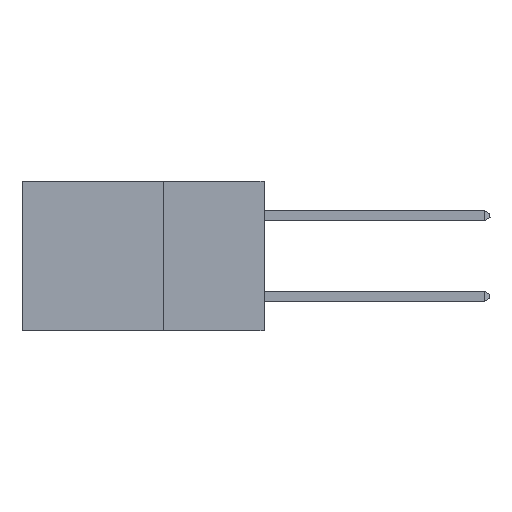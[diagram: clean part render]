
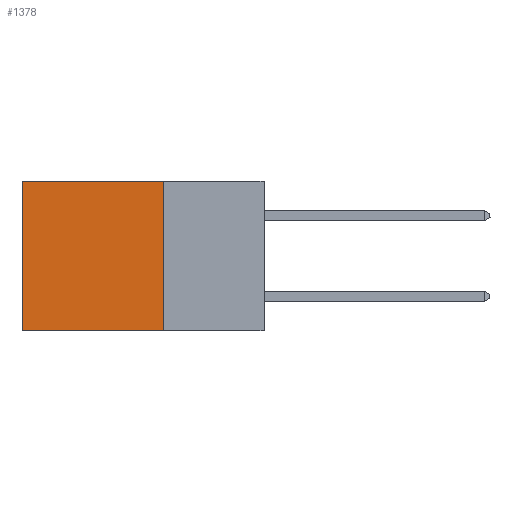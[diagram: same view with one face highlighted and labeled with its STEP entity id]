
A CAD part, left-side view. The second image highlights one B-rep face of the part: STEP entity #1378.
In plain terms, the highlighted planar face has unit normal (-1, 0, 0).
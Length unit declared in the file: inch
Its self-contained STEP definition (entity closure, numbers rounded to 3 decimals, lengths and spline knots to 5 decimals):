
#1378 = ADVANCED_FACE ( 'NONE', ( #26343 ), #22213, .F. ) ;
#2593 = CARTESIAN_POINT ( 'NONE',  ( 0.298, 0.25, 0. ) ) ;
#2702 = CARTESIAN_POINT ( 'NONE',  ( 0.298, 0.6, 0. ) ) ;
#2785 = LINE ( 'NONE', #24561, #25911 ) ;
#4151 = EDGE_CURVE ( 'NONE', #14430, #20718, #12649, .T. ) ;
#5920 = CARTESIAN_POINT ( 'NONE',  ( 0.298, 0.25, -0.37 ) ) ;
#7067 = EDGE_LOOP ( 'NONE', ( #11664, #24515, #17711, #7197 ) ) ;
#7197 = ORIENTED_EDGE ( 'NONE', *, *, #4151, .T. ) ;
#9749 = DIRECTION ( 'NONE',  ( 0., 1., 0. ) ) ;
#10123 = CARTESIAN_POINT ( 'NONE',  ( 0.298, 0.6, -0.37 ) ) ;
#10421 = DIRECTION ( 'NONE',  ( 0., 0., -1. ) ) ;
#10513 = CARTESIAN_POINT ( 'NONE',  ( 0.298, 0.25, 0. ) ) ;
#11664 = ORIENTED_EDGE ( 'NONE', *, *, #12083, .T. ) ;
#11986 = VECTOR ( 'NONE', #10421, 39.37008 ) ;
#12083 = EDGE_CURVE ( 'NONE', #20718, #16636, #14701, .T. ) ;
#12649 = LINE ( 'NONE', #19894, #18482 ) ;
#14430 = VERTEX_POINT ( 'NONE', #23888 ) ;
#14701 = LINE ( 'NONE', #2702, #11986 ) ;
#15027 = AXIS2_PLACEMENT_3D ( 'NONE', #2593, #22325, #19606 ) ;
#15712 = DIRECTION ( 'NONE',  ( 0., 0., -1. ) ) ;
#16636 = VERTEX_POINT ( 'NONE', #10123 ) ;
#17711 = ORIENTED_EDGE ( 'NONE', *, *, #23667, .F. ) ;
#17838 = CARTESIAN_POINT ( 'NONE',  ( 0.298, 0.6, 0. ) ) ;
#18482 = VECTOR ( 'NONE', #27424, 39.37008 ) ;
#19606 = DIRECTION ( 'NONE',  ( 0., 0., -1. ) ) ;
#19894 = CARTESIAN_POINT ( 'NONE',  ( 0.298, 0.25, 0. ) ) ;
#20718 = VERTEX_POINT ( 'NONE', #17838 ) ;
#22213 = PLANE ( 'NONE',  #15027 ) ;
#22325 = DIRECTION ( 'NONE',  ( 1., 0., 0. ) ) ;
#22479 = LINE ( 'NONE', #10513, #25187 ) ;
#23401 = VERTEX_POINT ( 'NONE', #5920 ) ;
#23667 = EDGE_CURVE ( 'NONE', #14430, #23401, #22479, .T. ) ;
#23888 = CARTESIAN_POINT ( 'NONE',  ( 0.298, 0.25, 0. ) ) ;
#24515 = ORIENTED_EDGE ( 'NONE', *, *, #30078, .F. ) ;
#24561 = CARTESIAN_POINT ( 'NONE',  ( 0.298, 0.25, -0.37 ) ) ;
#25187 = VECTOR ( 'NONE', #15712, 39.37008 ) ;
#25911 = VECTOR ( 'NONE', #9749, 39.37008 ) ;
#26343 = FACE_OUTER_BOUND ( 'NONE', #7067, .T. ) ;
#27424 = DIRECTION ( 'NONE',  ( 0., 1., 0. ) ) ;
#30078 = EDGE_CURVE ( 'NONE', #23401, #16636, #2785, .T. ) ;
